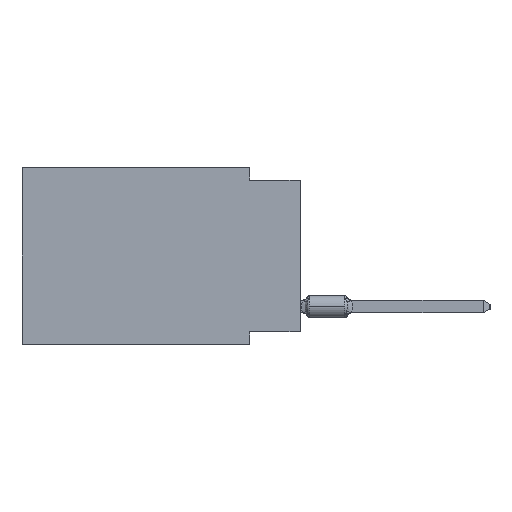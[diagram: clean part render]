
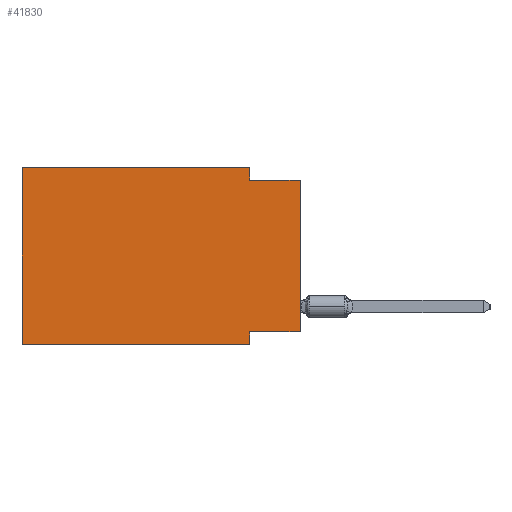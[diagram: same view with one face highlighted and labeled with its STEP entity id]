
A CAD part, left-side view. The second image highlights one B-rep face of the part: STEP entity #41830.
In plain terms, the highlighted planar face has unit normal (-1, 0, 0).
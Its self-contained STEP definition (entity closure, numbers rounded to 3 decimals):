
#278 = VECTOR ( 'NONE', #29490, 1000. ) ;
#353 = AXIS2_PLACEMENT_3D ( 'NONE', #49408, #28883, #54096 ) ;
#1268 = ORIENTED_EDGE ( 'NONE', *, *, #32614, .F. ) ;
#1415 = VECTOR ( 'NONE', #7292, 1000. ) ;
#5478 = CARTESIAN_POINT ( 'NONE',  ( 0., 2.54, 0. ) ) ;
#7220 = PLANE ( 'NONE',  #353 ) ;
#7292 = DIRECTION ( 'NONE',  ( 0., -1., 0. ) ) ;
#7841 = VECTOR ( 'NONE', #33043, 1000. ) ;
#7889 = ORIENTED_EDGE ( 'NONE', *, *, #13430, .T. ) ;
#8366 = CARTESIAN_POINT ( 'NONE',  ( 0., 0., -8.255 ) ) ;
#9362 = VERTEX_POINT ( 'NONE', #46988 ) ;
#9891 = CARTESIAN_POINT ( 'NONE',  ( 0., 2.54, -8.255 ) ) ;
#11761 = VERTEX_POINT ( 'NONE', #5478 ) ;
#12880 = CARTESIAN_POINT ( 'NONE',  ( 0., 2.54, -8.89 ) ) ;
#13194 = VECTOR ( 'NONE', #34485, 1000. ) ;
#13430 = EDGE_CURVE ( 'NONE', #38173, #53736, #23741, .T. ) ;
#13861 = EDGE_CURVE ( 'NONE', #21901, #22467, #44250, .T. ) ;
#14431 = ORIENTED_EDGE ( 'NONE', *, *, #40804, .F. ) ;
#15247 = VECTOR ( 'NONE', #15730, 1000. ) ;
#15395 = CARTESIAN_POINT ( 'NONE',  ( 0., 13.97, -8.89 ) ) ;
#15730 = DIRECTION ( 'NONE',  ( 0., 0., 1. ) ) ;
#15873 = VERTEX_POINT ( 'NONE', #9891 ) ;
#18292 = EDGE_CURVE ( 'NONE', #33739, #15873, #37140, .T. ) ;
#19162 = ORIENTED_EDGE ( 'NONE', *, *, #47826, .F. ) ;
#19545 = EDGE_LOOP ( 'NONE', ( #22652, #31641, #36593, #14431, #1268, #7889, #19162, #30910 ) ) ;
#21203 = CARTESIAN_POINT ( 'NONE',  ( 0., 2.54, -0.635 ) ) ;
#21367 = DIRECTION ( 'NONE',  ( 0., 0., -1. ) ) ;
#21888 = CARTESIAN_POINT ( 'NONE',  ( 0., 2.54, 0. ) ) ;
#21901 = VERTEX_POINT ( 'NONE', #21203 ) ;
#22467 = VERTEX_POINT ( 'NONE', #39713 ) ;
#22652 = ORIENTED_EDGE ( 'NONE', *, *, #23398, .T. ) ;
#23398 = EDGE_CURVE ( 'NONE', #33739, #22467, #44249, .T. ) ;
#23420 = DIRECTION ( 'NONE',  ( 0., -1., 0. ) ) ;
#23741 = LINE ( 'NONE', #40185, #1415 ) ;
#26524 = LINE ( 'NONE', #21888, #13194 ) ;
#28883 = DIRECTION ( 'NONE',  ( 1., 0., 0. ) ) ;
#29490 = DIRECTION ( 'NONE',  ( 0., -1., 0. ) ) ;
#30910 = ORIENTED_EDGE ( 'NONE', *, *, #18292, .F. ) ;
#31641 = ORIENTED_EDGE ( 'NONE', *, *, #13861, .F. ) ;
#32614 = EDGE_CURVE ( 'NONE', #38173, #9362, #45235, .T. ) ;
#33043 = DIRECTION ( 'NONE',  ( 0., 1., 0. ) ) ;
#33739 = VERTEX_POINT ( 'NONE', #44295 ) ;
#33869 = CARTESIAN_POINT ( 'NONE',  ( 0., 13.97, 0. ) ) ;
#34485 = DIRECTION ( 'NONE',  ( 0., 0., -1. ) ) ;
#35891 = CARTESIAN_POINT ( 'NONE',  ( 0., 2.54, -8.89 ) ) ;
#36593 = ORIENTED_EDGE ( 'NONE', *, *, #50618, .F. ) ;
#36842 = CARTESIAN_POINT ( 'NONE',  ( 0., 0., 0. ) ) ;
#37010 = CARTESIAN_POINT ( 'NONE',  ( 0., 13.97, 0. ) ) ;
#37140 = LINE ( 'NONE', #8366, #7841 ) ;
#38173 = VERTEX_POINT ( 'NONE', #15395 ) ;
#38629 = LINE ( 'NONE', #12880, #40229 ) ;
#39713 = CARTESIAN_POINT ( 'NONE',  ( 0., 0., -0.635 ) ) ;
#39953 = VECTOR ( 'NONE', #23420, 1000. ) ;
#40185 = CARTESIAN_POINT ( 'NONE',  ( 0., 13.97, -8.89 ) ) ;
#40229 = VECTOR ( 'NONE', #21367, 1000. ) ;
#40804 = EDGE_CURVE ( 'NONE', #9362, #11761, #45929, .T. ) ;
#41830 = ADVANCED_FACE ( 'NONE', ( #45033 ), #7220, .F. ) ;
#44249 = LINE ( 'NONE', #36842, #15247 ) ;
#44250 = LINE ( 'NONE', #53014, #39953 ) ;
#44295 = CARTESIAN_POINT ( 'NONE',  ( 0., 0., -8.255 ) ) ;
#45033 = FACE_OUTER_BOUND ( 'NONE', #19545, .T. ) ;
#45235 = LINE ( 'NONE', #37010, #51886 ) ;
#45929 = LINE ( 'NONE', #33869, #278 ) ;
#46988 = CARTESIAN_POINT ( 'NONE',  ( 0., 13.97, 0. ) ) ;
#47826 = EDGE_CURVE ( 'NONE', #15873, #53736, #38629, .T. ) ;
#49408 = CARTESIAN_POINT ( 'NONE',  ( 0., 13.97, 0. ) ) ;
#50618 = EDGE_CURVE ( 'NONE', #11761, #21901, #26524, .T. ) ;
#51886 = VECTOR ( 'NONE', #53726, 1000. ) ;
#53014 = CARTESIAN_POINT ( 'NONE',  ( 0., 0., -0.635 ) ) ;
#53726 = DIRECTION ( 'NONE',  ( 0., 0., 1. ) ) ;
#53736 = VERTEX_POINT ( 'NONE', #35891 ) ;
#54096 = DIRECTION ( 'NONE',  ( 0., 0., -1. ) ) ;
